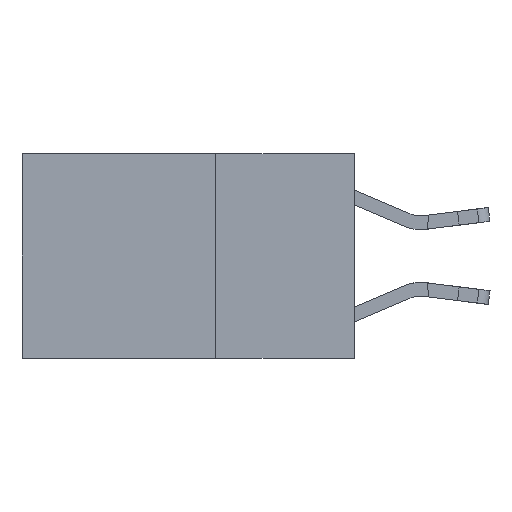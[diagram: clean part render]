
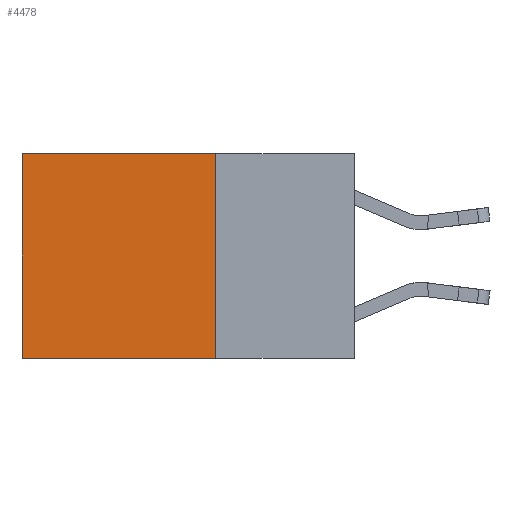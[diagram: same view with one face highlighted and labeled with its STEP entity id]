
A CAD part, left-side view. The second image highlights one B-rep face of the part: STEP entity #4478.
In plain terms, the highlighted planar face has unit normal (-1, 0, 0).
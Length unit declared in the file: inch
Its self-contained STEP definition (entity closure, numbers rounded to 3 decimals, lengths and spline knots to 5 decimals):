
#813 = CARTESIAN_POINT ( 'NONE',  ( 0.2625, 0.6, 0. ) ) ;
#844 = AXIS2_PLACEMENT_3D ( 'NONE', #8647, #11447, #4611 ) ;
#1027 = DIRECTION ( 'NONE',  ( 0., 0., -1. ) ) ;
#1139 = PLANE ( 'NONE',  #844 ) ;
#1362 = VECTOR ( 'NONE', #1977, 39.37008 ) ;
#1854 = VECTOR ( 'NONE', #1027, 39.37008 ) ;
#1977 = DIRECTION ( 'NONE',  ( 0., 0., -1. ) ) ;
#1989 = ORIENTED_EDGE ( 'NONE', *, *, #6988, .F. ) ;
#3136 = EDGE_CURVE ( 'NONE', #14682, #5386, #7561, .T. ) ;
#3899 = LINE ( 'NONE', #5142, #10314 ) ;
#4444 = LINE ( 'NONE', #7653, #1362 ) ;
#4478 = ADVANCED_FACE ( 'NONE', ( #10207 ), #1139, .F. ) ;
#4611 = DIRECTION ( 'NONE',  ( 0., 0., -1. ) ) ;
#5028 = ORIENTED_EDGE ( 'NONE', *, *, #7801, .F. ) ;
#5142 = CARTESIAN_POINT ( 'NONE',  ( 0.2625, 0.25, -0.37 ) ) ;
#5386 = VERTEX_POINT ( 'NONE', #14118 ) ;
#5709 = EDGE_LOOP ( 'NONE', ( #7693, #1989, #5028, #8040 ) ) ;
#6988 = EDGE_CURVE ( 'NONE', #9274, #5386, #3899, .T. ) ;
#7561 = LINE ( 'NONE', #813, #1854 ) ;
#7653 = CARTESIAN_POINT ( 'NONE',  ( 0.2625, 0.25, 0. ) ) ;
#7693 = ORIENTED_EDGE ( 'NONE', *, *, #3136, .T. ) ;
#7801 = EDGE_CURVE ( 'NONE', #14499, #9274, #4444, .T. ) ;
#8040 = ORIENTED_EDGE ( 'NONE', *, *, #12373, .T. ) ;
#8593 = VECTOR ( 'NONE', #14091, 39.37008 ) ;
#8647 = CARTESIAN_POINT ( 'NONE',  ( 0.2625, 0.25, 0. ) ) ;
#9274 = VERTEX_POINT ( 'NONE', #12067 ) ;
#10207 = FACE_OUTER_BOUND ( 'NONE', #5709, .T. ) ;
#10314 = VECTOR ( 'NONE', #14271, 39.37008 ) ;
#11447 = DIRECTION ( 'NONE',  ( 1., 0., 0. ) ) ;
#11638 = LINE ( 'NONE', #11753, #8593 ) ;
#11753 = CARTESIAN_POINT ( 'NONE',  ( 0.2625, 0.25, 0. ) ) ;
#12067 = CARTESIAN_POINT ( 'NONE',  ( 0.2625, 0.25, -0.37 ) ) ;
#12117 = CARTESIAN_POINT ( 'NONE',  ( 0.2625, 0.25, 0. ) ) ;
#12373 = EDGE_CURVE ( 'NONE', #14499, #14682, #11638, .T. ) ;
#14091 = DIRECTION ( 'NONE',  ( 0., 1., 0. ) ) ;
#14118 = CARTESIAN_POINT ( 'NONE',  ( 0.2625, 0.6, -0.37 ) ) ;
#14271 = DIRECTION ( 'NONE',  ( 0., 1., 0. ) ) ;
#14499 = VERTEX_POINT ( 'NONE', #12117 ) ;
#14676 = CARTESIAN_POINT ( 'NONE',  ( 0.2625, 0.6, 0. ) ) ;
#14682 = VERTEX_POINT ( 'NONE', #14676 ) ;
